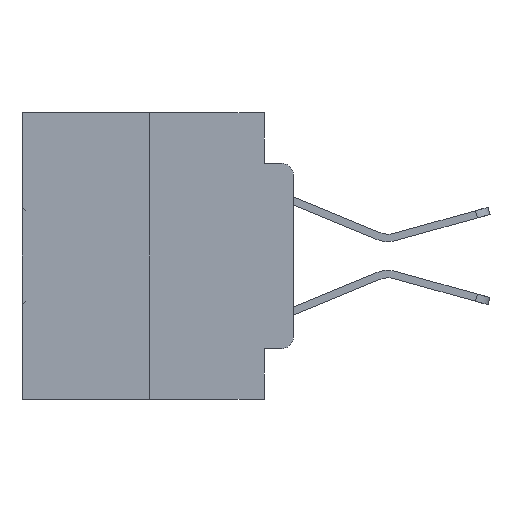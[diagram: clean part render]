
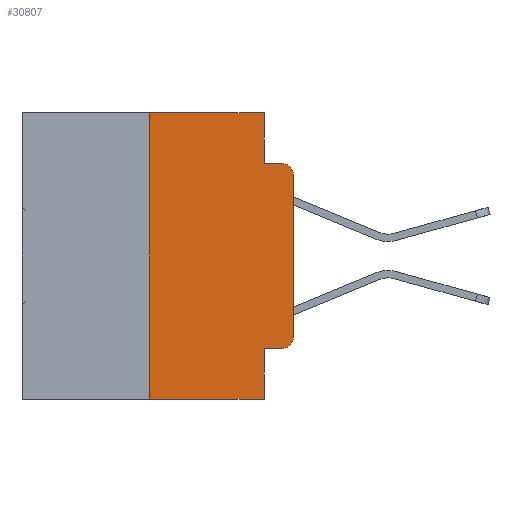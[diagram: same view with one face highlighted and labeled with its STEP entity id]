
A CAD part, left-side view. The second image highlights one B-rep face of the part: STEP entity #30807.
In plain terms, the highlighted planar face has unit normal (-1, 0, 0).
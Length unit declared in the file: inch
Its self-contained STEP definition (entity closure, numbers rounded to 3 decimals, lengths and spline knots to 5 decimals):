
#729 = VERTEX_POINT ( 'NONE', #1233 ) ;
#877 = VERTEX_POINT ( 'NONE', #31525 ) ;
#1233 = CARTESIAN_POINT ( 'NONE',  ( 0., 0.051, -0.5 ) ) ;
#1967 = CIRCLE ( 'NONE', #29384, 0.02 ) ;
#2224 = VERTEX_POINT ( 'NONE', #9114 ) ;
#2497 = EDGE_CURVE ( 'NONE', #7070, #877, #6862, .T. ) ;
#3794 = CARTESIAN_POINT ( 'NONE',  ( 0., 0.02, -0.3915 ) ) ;
#3821 = DIRECTION ( 'NONE',  ( 0., -1., 0. ) ) ;
#4338 = VERTEX_POINT ( 'NONE', #26001 ) ;
#4529 = EDGE_CURVE ( 'NONE', #4338, #729, #22478, .T. ) ;
#4963 = CARTESIAN_POINT ( 'NONE',  ( 0., 0.051, -0.0885 ) ) ;
#5092 = VECTOR ( 'NONE', #3821, 39.37008 ) ;
#6274 = DIRECTION ( 'NONE',  ( 0., 0., -1. ) ) ;
#6311 = DIRECTION ( 'NONE',  ( 0., -1., 0. ) ) ;
#6862 = LINE ( 'NONE', #14345, #19437 ) ;
#7007 = CARTESIAN_POINT ( 'NONE',  ( 0., 0.051, 0. ) ) ;
#7070 = VERTEX_POINT ( 'NONE', #11578 ) ;
#8341 = DIRECTION ( 'NONE',  ( 1., 0., 0. ) ) ;
#8634 = CARTESIAN_POINT ( 'NONE',  ( 0., 0.02, -0.1085 ) ) ;
#8679 = VERTEX_POINT ( 'NONE', #10807 ) ;
#8807 = AXIS2_PLACEMENT_3D ( 'NONE', #8634, #26229, #11173 ) ;
#9114 = CARTESIAN_POINT ( 'NONE',  ( 0., 0., -0.1085 ) ) ;
#9540 = CARTESIAN_POINT ( 'NONE',  ( 0., 0.02, -0.4115 ) ) ;
#9570 = EDGE_CURVE ( 'NONE', #12381, #12205, #1967, .T. ) ;
#9785 = ORIENTED_EDGE ( 'NONE', *, *, #28170, .F. ) ;
#9822 = ORIENTED_EDGE ( 'NONE', *, *, #27236, .T. ) ;
#10807 = CARTESIAN_POINT ( 'NONE',  ( 0., 0.02, -0.0885 ) ) ;
#11173 = DIRECTION ( 'NONE',  ( 0., 0., -1. ) ) ;
#11395 = ORIENTED_EDGE ( 'NONE', *, *, #2497, .F. ) ;
#11578 = CARTESIAN_POINT ( 'NONE',  ( 0., 0.25, -0.5 ) ) ;
#11984 = VECTOR ( 'NONE', #27557, 39.37008 ) ;
#12205 = VERTEX_POINT ( 'NONE', #13854 ) ;
#12240 = CARTESIAN_POINT ( 'NONE',  ( 0., 0., 0. ) ) ;
#12381 = VERTEX_POINT ( 'NONE', #9540 ) ;
#12514 = LINE ( 'NONE', #26290, #5092 ) ;
#13086 = CARTESIAN_POINT ( 'NONE',  ( 0., 0.051, -0.0885 ) ) ;
#13603 = LINE ( 'NONE', #18275, #26984 ) ;
#13784 = ORIENTED_EDGE ( 'NONE', *, *, #4529, .F. ) ;
#13854 = CARTESIAN_POINT ( 'NONE',  ( 0., 0., -0.3915 ) ) ;
#14211 = LINE ( 'NONE', #29368, #20130 ) ;
#14345 = CARTESIAN_POINT ( 'NONE',  ( 0., 0.25, 0. ) ) ;
#15826 = CARTESIAN_POINT ( 'NONE',  ( 0., 0.473, 0. ) ) ;
#17503 = VERTEX_POINT ( 'NONE', #22903 ) ;
#18275 = CARTESIAN_POINT ( 'NONE',  ( 0., 0.051, 0. ) ) ;
#18457 = AXIS2_PLACEMENT_3D ( 'NONE', #15826, #8341, #25931 ) ;
#19280 = EDGE_CURVE ( 'NONE', #877, #17503, #12514, .T. ) ;
#19437 = VECTOR ( 'NONE', #31360, 39.37008 ) ;
#19679 = VERTEX_POINT ( 'NONE', #13086 ) ;
#19851 = DIRECTION ( 'NONE',  ( 0., 0., 1. ) ) ;
#19870 = CIRCLE ( 'NONE', #8807, 0.02 ) ;
#20034 = ORIENTED_EDGE ( 'NONE', *, *, #28787, .T. ) ;
#20130 = VECTOR ( 'NONE', #24480, 39.37008 ) ;
#20346 = VECTOR ( 'NONE', #6311, 39.37008 ) ;
#20401 = DIRECTION ( 'NONE',  ( 0., 0., -1. ) ) ;
#20631 = LINE ( 'NONE', #12240, #26502 ) ;
#20724 = ORIENTED_EDGE ( 'NONE', *, *, #19280, .F. ) ;
#21126 = LINE ( 'NONE', #26416, #20346 ) ;
#21340 = DIRECTION ( 'NONE',  ( -1., 0., 0. ) ) ;
#21470 = EDGE_CURVE ( 'NONE', #2224, #8679, #19870, .T. ) ;
#22478 = LINE ( 'NONE', #7007, #28359 ) ;
#22903 = CARTESIAN_POINT ( 'NONE',  ( 0., 0.051, 0. ) ) ;
#23442 = EDGE_CURVE ( 'NONE', #4338, #12381, #14211, .T. ) ;
#24480 = DIRECTION ( 'NONE',  ( 0., -1., 0. ) ) ;
#25298 = ORIENTED_EDGE ( 'NONE', *, *, #23442, .T. ) ;
#25722 = DIRECTION ( 'NONE',  ( 0., 0., -1. ) ) ;
#25821 = PLANE ( 'NONE',  #18457 ) ;
#25931 = DIRECTION ( 'NONE',  ( 0., 0., -1. ) ) ;
#26001 = CARTESIAN_POINT ( 'NONE',  ( 0., 0.051, -0.4115 ) ) ;
#26151 = LINE ( 'NONE', #4963, #11984 ) ;
#26229 = DIRECTION ( 'NONE',  ( -1., 0., 0. ) ) ;
#26290 = CARTESIAN_POINT ( 'NONE',  ( 0., 0.473, 0. ) ) ;
#26416 = CARTESIAN_POINT ( 'NONE',  ( 0., 0.473, -0.5 ) ) ;
#26502 = VECTOR ( 'NONE', #19851, 39.37008 ) ;
#26731 = ORIENTED_EDGE ( 'NONE', *, *, #27696, .F. ) ;
#26834 = FACE_OUTER_BOUND ( 'NONE', #30572, .T. ) ;
#26984 = VECTOR ( 'NONE', #25722, 39.37008 ) ;
#27236 = EDGE_CURVE ( 'NONE', #7070, #729, #21126, .T. ) ;
#27557 = DIRECTION ( 'NONE',  ( 0., -1., 0. ) ) ;
#27696 = EDGE_CURVE ( 'NONE', #17503, #19679, #13603, .T. ) ;
#27888 = ORIENTED_EDGE ( 'NONE', *, *, #21470, .T. ) ;
#28170 = EDGE_CURVE ( 'NONE', #19679, #8679, #26151, .T. ) ;
#28359 = VECTOR ( 'NONE', #20401, 39.37008 ) ;
#28787 = EDGE_CURVE ( 'NONE', #12205, #2224, #20631, .T. ) ;
#29368 = CARTESIAN_POINT ( 'NONE',  ( 0., 0.051, -0.4115 ) ) ;
#29384 = AXIS2_PLACEMENT_3D ( 'NONE', #3794, #21340, #6274 ) ;
#30572 = EDGE_LOOP ( 'NONE', ( #20034, #27888, #9785, #26731, #20724, #11395, #9822, #13784, #25298, #30995 ) ) ;
#30807 = ADVANCED_FACE ( 'NONE', ( #26834 ), #25821, .F. ) ;
#30995 = ORIENTED_EDGE ( 'NONE', *, *, #9570, .T. ) ;
#31360 = DIRECTION ( 'NONE',  ( 0., 0., 1. ) ) ;
#31525 = CARTESIAN_POINT ( 'NONE',  ( 0., 0.25, 0. ) ) ;
